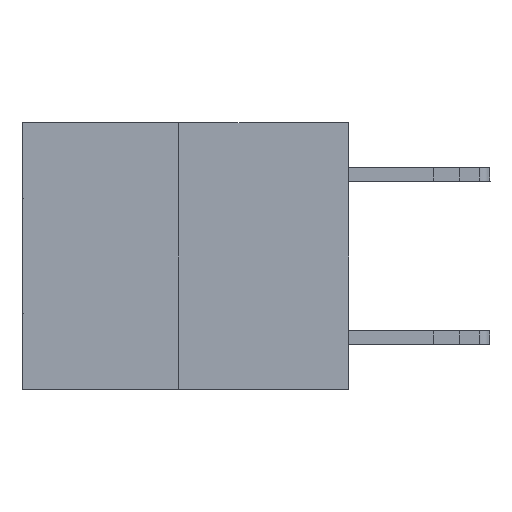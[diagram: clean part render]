
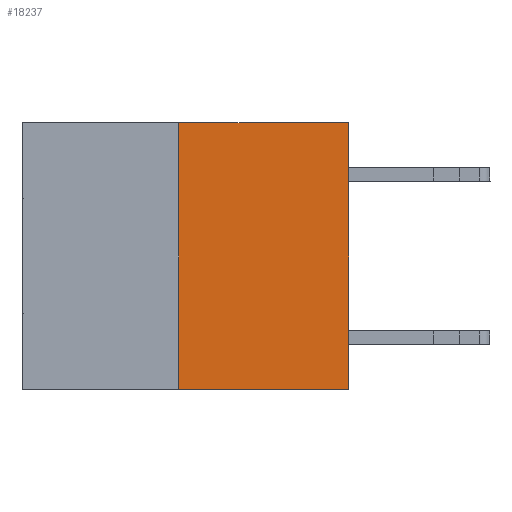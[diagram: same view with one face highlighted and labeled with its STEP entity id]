
A CAD part, left-side view. The second image highlights one B-rep face of the part: STEP entity #18237.
In plain terms, the highlighted planar face has unit normal (-1, 0, 0).
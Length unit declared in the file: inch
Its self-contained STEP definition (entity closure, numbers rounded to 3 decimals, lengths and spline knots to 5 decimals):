
#519 = CARTESIAN_POINT ( 'NONE',  ( 0., 0.312, -0.49 ) ) ;
#2288 = DIRECTION ( 'NONE',  ( 0., 0., -1. ) ) ;
#3938 = LINE ( 'NONE', #11324, #18057 ) ;
#4853 = CARTESIAN_POINT ( 'NONE',  ( 0., 0.312, 0. ) ) ;
#4862 = VECTOR ( 'NONE', #24917, 39.37008 ) ;
#6038 = LINE ( 'NONE', #6590, #11410 ) ;
#6590 = CARTESIAN_POINT ( 'NONE',  ( 0., 0., 0. ) ) ;
#7143 = FACE_OUTER_BOUND ( 'NONE', #27276, .T. ) ;
#9784 = DIRECTION ( 'NONE',  ( 1., 0., 0. ) ) ;
#10095 = AXIS2_PLACEMENT_3D ( 'NONE', #31658, #9784, #2288 ) ;
#10251 = CARTESIAN_POINT ( 'NONE',  ( 0., 0.6, -0.49 ) ) ;
#11204 = EDGE_CURVE ( 'NONE', #25036, #23007, #30173, .T. ) ;
#11324 = CARTESIAN_POINT ( 'NONE',  ( 0., 0.6, 0. ) ) ;
#11410 = VECTOR ( 'NONE', #14115, 39.37008 ) ;
#13151 = ORIENTED_EDGE ( 'NONE', *, *, #29415, .F. ) ;
#13561 = CARTESIAN_POINT ( 'NONE',  ( 0., 0., 0. ) ) ;
#14115 = DIRECTION ( 'NONE',  ( 0., 0., 1. ) ) ;
#15640 = VECTOR ( 'NONE', #19914, 39.37008 ) ;
#15652 = VERTEX_POINT ( 'NONE', #13561 ) ;
#18057 = VECTOR ( 'NONE', #23403, 39.37008 ) ;
#18237 = ADVANCED_FACE ( 'NONE', ( #7143 ), #27230, .F. ) ;
#19484 = CARTESIAN_POINT ( 'NONE',  ( 0., 0., -0.49 ) ) ;
#19914 = DIRECTION ( 'NONE',  ( 0., 0., 1. ) ) ;
#20491 = CARTESIAN_POINT ( 'NONE',  ( 0., 0.312, -0.49 ) ) ;
#22135 = LINE ( 'NONE', #519, #15640 ) ;
#23007 = VERTEX_POINT ( 'NONE', #19484 ) ;
#23403 = DIRECTION ( 'NONE',  ( 0., -1., 0. ) ) ;
#24534 = ORIENTED_EDGE ( 'NONE', *, *, #24691, .F. ) ;
#24691 = EDGE_CURVE ( 'NONE', #25036, #27726, #22135, .T. ) ;
#24711 = ORIENTED_EDGE ( 'NONE', *, *, #30740, .T. ) ;
#24917 = DIRECTION ( 'NONE',  ( 0., -1., 0. ) ) ;
#25036 = VERTEX_POINT ( 'NONE', #20491 ) ;
#26913 = ORIENTED_EDGE ( 'NONE', *, *, #11204, .T. ) ;
#27230 = PLANE ( 'NONE',  #10095 ) ;
#27276 = EDGE_LOOP ( 'NONE', ( #24534, #26913, #24711, #13151 ) ) ;
#27726 = VERTEX_POINT ( 'NONE', #4853 ) ;
#29415 = EDGE_CURVE ( 'NONE', #27726, #15652, #3938, .T. ) ;
#30173 = LINE ( 'NONE', #10251, #4862 ) ;
#30740 = EDGE_CURVE ( 'NONE', #23007, #15652, #6038, .T. ) ;
#31658 = CARTESIAN_POINT ( 'NONE',  ( 0., 0.6, 0. ) ) ;
